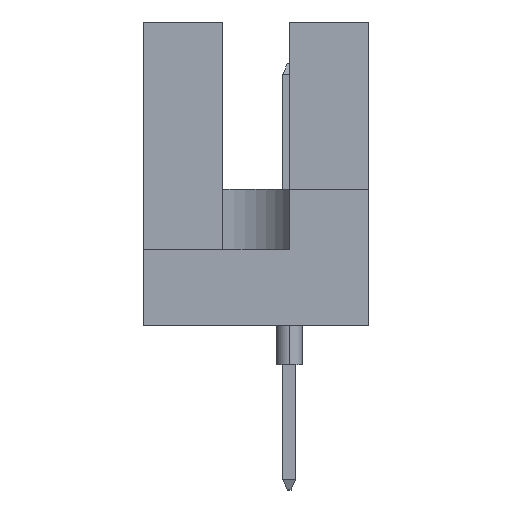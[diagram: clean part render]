
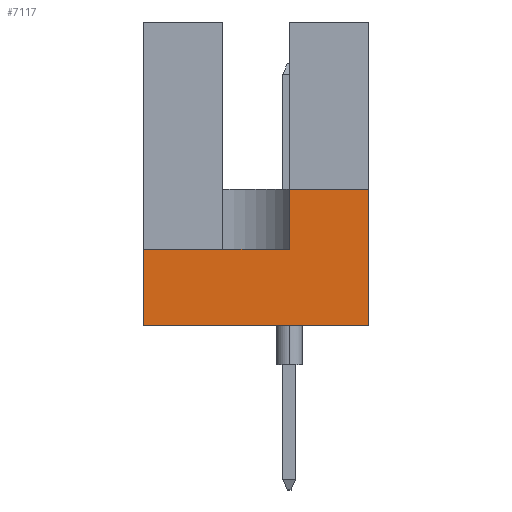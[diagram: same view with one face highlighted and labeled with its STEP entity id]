
A CAD part, left-side view. The second image highlights one B-rep face of the part: STEP entity #7117.
In plain terms, the highlighted planar face has unit normal (-1, 0, 0).
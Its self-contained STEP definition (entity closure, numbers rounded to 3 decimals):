
#405 = ORIENTED_EDGE ( 'NONE', *, *, #6541, .T. ) ;
#495 = CARTESIAN_POINT ( 'NONE',  ( -47.5, 4.3, 0. ) ) ;
#588 = VERTEX_POINT ( 'NONE', #8308 ) ;
#604 = ORIENTED_EDGE ( 'NONE', *, *, #11459, .F. ) ;
#785 = AXIS2_PLACEMENT_3D ( 'NONE', #1747, #9926, #3509 ) ;
#1039 = CARTESIAN_POINT ( 'NONE',  ( -47.5, -4.3, 5.2 ) ) ;
#1232 = EDGE_LOOP ( 'NONE', ( #604, #6281, #10888, #10093, #405, #11224 ) ) ;
#1727 = VECTOR ( 'NONE', #3524, 1000. ) ;
#1747 = CARTESIAN_POINT ( 'NONE',  ( -47.5, 4.3, 11.6 ) ) ;
#1750 = LINE ( 'NONE', #6364, #5822 ) ;
#1864 = EDGE_CURVE ( 'NONE', #10243, #4706, #2070, .T. ) ;
#2070 = LINE ( 'NONE', #2247, #6794 ) ;
#2125 = DIRECTION ( 'NONE',  ( 0., -1., 0. ) ) ;
#2247 = CARTESIAN_POINT ( 'NONE',  ( -47.5, -4.3, 11.6 ) ) ;
#2494 = CARTESIAN_POINT ( 'NONE',  ( -47.5, -1.27, 2.9 ) ) ;
#2689 = FACE_OUTER_BOUND ( 'NONE', #1232, .T. ) ;
#2856 = PLANE ( 'NONE',  #785 ) ;
#3456 = VECTOR ( 'NONE', #8984, 1000. ) ;
#3509 = DIRECTION ( 'NONE',  ( 0., 0., -1. ) ) ;
#3524 = DIRECTION ( 'NONE',  ( 0., 0., -1. ) ) ;
#3793 = DIRECTION ( 'NONE',  ( 0., 1., 0. ) ) ;
#4706 = VERTEX_POINT ( 'NONE', #5526 ) ;
#4935 = LINE ( 'NONE', #495, #8276 ) ;
#5526 = CARTESIAN_POINT ( 'NONE',  ( -47.5, -4.3, 0. ) ) ;
#5808 = DIRECTION ( 'NONE',  ( 0., 0., -1. ) ) ;
#5822 = VECTOR ( 'NONE', #3793, 1000. ) ;
#6281 = ORIENTED_EDGE ( 'NONE', *, *, #7778, .T. ) ;
#6364 = CARTESIAN_POINT ( 'NONE',  ( -47.5, 4.3, 2.9 ) ) ;
#6541 = EDGE_CURVE ( 'NONE', #588, #4706, #4935, .T. ) ;
#6755 = DIRECTION ( 'NONE',  ( 0., 0., -1. ) ) ;
#6794 = VECTOR ( 'NONE', #5808, 1000. ) ;
#6965 = CARTESIAN_POINT ( 'NONE',  ( -47.5, -1.27, 19.02 ) ) ;
#7117 = ADVANCED_FACE ( 'NONE', ( #2689 ), #2856, .F. ) ;
#7778 = EDGE_CURVE ( 'NONE', #11348, #11458, #11535, .T. ) ;
#7813 = CARTESIAN_POINT ( 'NONE',  ( -47.5, 4.3, 5.2 ) ) ;
#7992 = CARTESIAN_POINT ( 'NONE',  ( -47.5, -1.27, 5.2 ) ) ;
#8276 = VECTOR ( 'NONE', #2125, 1000. ) ;
#8308 = CARTESIAN_POINT ( 'NONE',  ( -47.5, 4.3, 0. ) ) ;
#8402 = CARTESIAN_POINT ( 'NONE',  ( -47.5, 4.3, 11.6 ) ) ;
#8436 = EDGE_CURVE ( 'NONE', #11458, #10842, #1750, .T. ) ;
#8475 = CARTESIAN_POINT ( 'NONE',  ( -47.5, 4.3, 2.9 ) ) ;
#8984 = DIRECTION ( 'NONE',  ( 0., -1., 0. ) ) ;
#9854 = EDGE_CURVE ( 'NONE', #10842, #588, #10392, .T. ) ;
#9926 = DIRECTION ( 'NONE',  ( 1., 0., 0. ) ) ;
#9961 = VECTOR ( 'NONE', #6755, 1000. ) ;
#10093 = ORIENTED_EDGE ( 'NONE', *, *, #9854, .T. ) ;
#10243 = VERTEX_POINT ( 'NONE', #1039 ) ;
#10392 = LINE ( 'NONE', #8402, #9961 ) ;
#10615 = LINE ( 'NONE', #7813, #3456 ) ;
#10842 = VERTEX_POINT ( 'NONE', #8475 ) ;
#10888 = ORIENTED_EDGE ( 'NONE', *, *, #8436, .T. ) ;
#11224 = ORIENTED_EDGE ( 'NONE', *, *, #1864, .F. ) ;
#11348 = VERTEX_POINT ( 'NONE', #7992 ) ;
#11458 = VERTEX_POINT ( 'NONE', #2494 ) ;
#11459 = EDGE_CURVE ( 'NONE', #11348, #10243, #10615, .T. ) ;
#11535 = LINE ( 'NONE', #6965, #1727 ) ;
